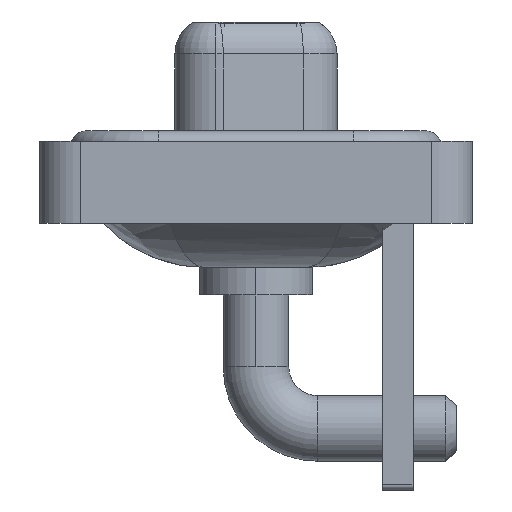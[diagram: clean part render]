
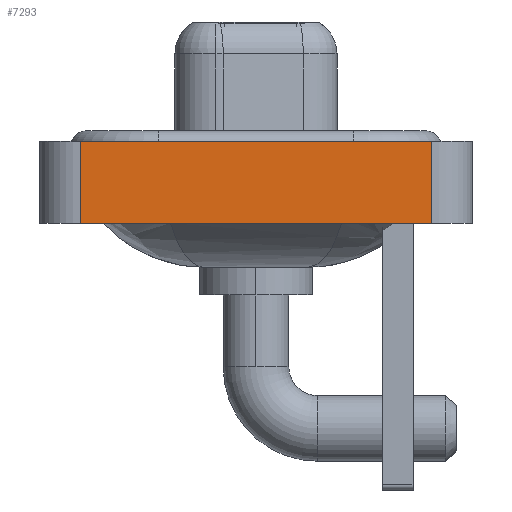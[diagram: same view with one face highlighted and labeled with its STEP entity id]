
A CAD part, left-side view. The second image highlights one B-rep face of the part: STEP entity #7293.
In plain terms, the highlighted planar face has unit normal (-1, 0, 0).
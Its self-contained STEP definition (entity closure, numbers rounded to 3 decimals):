
#55 = EDGE_LOOP ( 'NONE', ( #16683, #2137, #11150, #13816 ) ) ;
#473 = LINE ( 'NONE', #4875, #15700 ) ;
#480 = CARTESIAN_POINT ( 'NONE',  ( -7.35, -8.55, 0.4 ) ) ;
#1167 = VERTEX_POINT ( 'NONE', #8791 ) ;
#1272 = EDGE_CURVE ( 'NONE', #8070, #10456, #16125, .T. ) ;
#1595 = CARTESIAN_POINT ( 'NONE',  ( -7.35, -8.55, -3.6 ) ) ;
#2056 = DIRECTION ( 'NONE',  ( 0., 0., 1. ) ) ;
#2137 = ORIENTED_EDGE ( 'NONE', *, *, #12874, .F. ) ;
#4092 = CARTESIAN_POINT ( 'NONE',  ( -7.35, -8.55, -3.6 ) ) ;
#4709 = DIRECTION ( 'NONE',  ( 0., -1., 0. ) ) ;
#4875 = CARTESIAN_POINT ( 'NONE',  ( -7.35, 8.55, -3.6 ) ) ;
#5038 = VERTEX_POINT ( 'NONE', #12572 ) ;
#5556 = EDGE_CURVE ( 'NONE', #10456, #1167, #6719, .T. ) ;
#5794 = VECTOR ( 'NONE', #12153, 1000. ) ;
#6021 = AXIS2_PLACEMENT_3D ( 'NONE', #1595, #14055, #8079 ) ;
#6719 = LINE ( 'NONE', #13295, #10470 ) ;
#7293 = ADVANCED_FACE ( 'NONE', ( #8351 ), #16173, .T. ) ;
#8070 = VERTEX_POINT ( 'NONE', #16009 ) ;
#8079 = DIRECTION ( 'NONE',  ( 0., 0., 1. ) ) ;
#8351 = FACE_OUTER_BOUND ( 'NONE', #55, .T. ) ;
#8791 = CARTESIAN_POINT ( 'NONE',  ( -7.35, -8.55, 0.4 ) ) ;
#9859 = CARTESIAN_POINT ( 'NONE',  ( -7.35, -8.55, -3.6 ) ) ;
#10054 = VECTOR ( 'NONE', #4709, 1000. ) ;
#10456 = VERTEX_POINT ( 'NONE', #9859 ) ;
#10470 = VECTOR ( 'NONE', #12809, 1000. ) ;
#11093 = EDGE_CURVE ( 'NONE', #8070, #5038, #473, .T. ) ;
#11150 = ORIENTED_EDGE ( 'NONE', *, *, #11093, .F. ) ;
#12153 = DIRECTION ( 'NONE',  ( 0., -1., 0. ) ) ;
#12572 = CARTESIAN_POINT ( 'NONE',  ( -7.35, 8.55, 0.4 ) ) ;
#12809 = DIRECTION ( 'NONE',  ( 0., 0., 1. ) ) ;
#12874 = EDGE_CURVE ( 'NONE', #5038, #1167, #16732, .T. ) ;
#13295 = CARTESIAN_POINT ( 'NONE',  ( -7.35, -8.55, -3.6 ) ) ;
#13816 = ORIENTED_EDGE ( 'NONE', *, *, #1272, .T. ) ;
#14055 = DIRECTION ( 'NONE',  ( -1., 0., 0. ) ) ;
#15700 = VECTOR ( 'NONE', #2056, 1000. ) ;
#16009 = CARTESIAN_POINT ( 'NONE',  ( -7.35, 8.55, -3.6 ) ) ;
#16125 = LINE ( 'NONE', #4092, #5794 ) ;
#16173 = PLANE ( 'NONE',  #6021 ) ;
#16683 = ORIENTED_EDGE ( 'NONE', *, *, #5556, .T. ) ;
#16732 = LINE ( 'NONE', #480, #10054 ) ;
